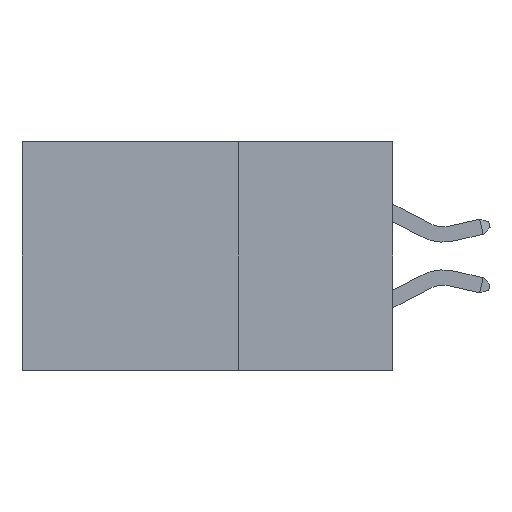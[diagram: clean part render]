
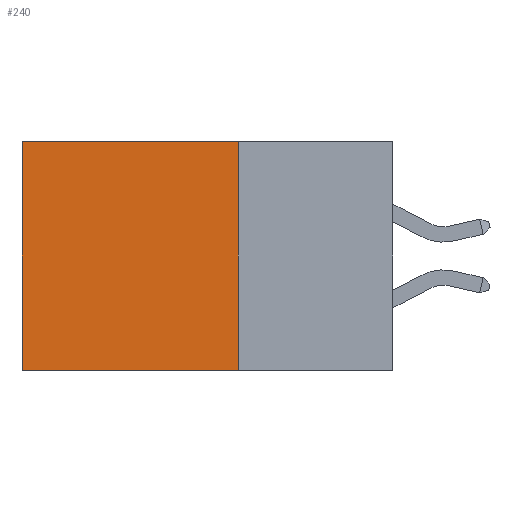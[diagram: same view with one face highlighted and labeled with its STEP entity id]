
A CAD part, left-side view. The second image highlights one B-rep face of the part: STEP entity #240.
In plain terms, the highlighted planar face has unit normal (-1, 0, 0).
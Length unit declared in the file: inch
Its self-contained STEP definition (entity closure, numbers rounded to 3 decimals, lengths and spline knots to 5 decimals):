
#116 = LINE ( 'NONE', #8964, #6563 ) ;
#240 = ADVANCED_FACE ( 'NONE', ( #7745 ), #2963, .F. ) ;
#363 = LINE ( 'NONE', #8911, #9792 ) ;
#667 = DIRECTION ( 'NONE',  ( 0., 0., -1. ) ) ;
#880 = CARTESIAN_POINT ( 'NONE',  ( 0.2875, 0.25, 0. ) ) ;
#993 = EDGE_CURVE ( 'NONE', #4801, #1453, #116, .T. ) ;
#1230 = ORIENTED_EDGE ( 'NONE', *, *, #5009, .T. ) ;
#1377 = EDGE_CURVE ( 'NONE', #4801, #2131, #6943, .T. ) ;
#1453 = VERTEX_POINT ( 'NONE', #8497 ) ;
#1530 = ORIENTED_EDGE ( 'NONE', *, *, #7189, .F. ) ;
#1556 = ORIENTED_EDGE ( 'NONE', *, *, #1377, .F. ) ;
#1631 = DIRECTION ( 'NONE',  ( 0., 1., 0. ) ) ;
#1652 = ORIENTED_EDGE ( 'NONE', *, *, #993, .T. ) ;
#2131 = VERTEX_POINT ( 'NONE', #5970 ) ;
#2398 = VECTOR ( 'NONE', #8949, 39.37008 ) ;
#2963 = PLANE ( 'NONE',  #4676 ) ;
#3145 = VECTOR ( 'NONE', #667, 39.37008 ) ;
#4456 = CARTESIAN_POINT ( 'NONE',  ( 0.2875, 0.25, 0. ) ) ;
#4562 = LINE ( 'NONE', #7018, #2398 ) ;
#4676 = AXIS2_PLACEMENT_3D ( 'NONE', #4456, #6911, #7834 ) ;
#4801 = VERTEX_POINT ( 'NONE', #8849 ) ;
#5009 = EDGE_CURVE ( 'NONE', #1453, #8933, #4562, .T. ) ;
#5560 = CARTESIAN_POINT ( 'NONE',  ( 0.2875, 0.6, -0.37 ) ) ;
#5970 = CARTESIAN_POINT ( 'NONE',  ( 0.2875, 0.25, -0.37 ) ) ;
#6144 = EDGE_LOOP ( 'NONE', ( #1230, #1530, #1556, #1652 ) ) ;
#6563 = VECTOR ( 'NONE', #7351, 39.37008 ) ;
#6911 = DIRECTION ( 'NONE',  ( 1., 0., 0. ) ) ;
#6943 = LINE ( 'NONE', #880, #3145 ) ;
#7018 = CARTESIAN_POINT ( 'NONE',  ( 0.2875, 0.6, 0. ) ) ;
#7189 = EDGE_CURVE ( 'NONE', #2131, #8933, #363, .T. ) ;
#7351 = DIRECTION ( 'NONE',  ( 0., 1., 0. ) ) ;
#7745 = FACE_OUTER_BOUND ( 'NONE', #6144, .T. ) ;
#7834 = DIRECTION ( 'NONE',  ( 0., 0., -1. ) ) ;
#8497 = CARTESIAN_POINT ( 'NONE',  ( 0.2875, 0.6, 0. ) ) ;
#8849 = CARTESIAN_POINT ( 'NONE',  ( 0.2875, 0.25, 0. ) ) ;
#8911 = CARTESIAN_POINT ( 'NONE',  ( 0.2875, 0.25, -0.37 ) ) ;
#8933 = VERTEX_POINT ( 'NONE', #5560 ) ;
#8949 = DIRECTION ( 'NONE',  ( 0., 0., -1. ) ) ;
#8964 = CARTESIAN_POINT ( 'NONE',  ( 0.2875, 0.25, 0. ) ) ;
#9792 = VECTOR ( 'NONE', #1631, 39.37008 ) ;
